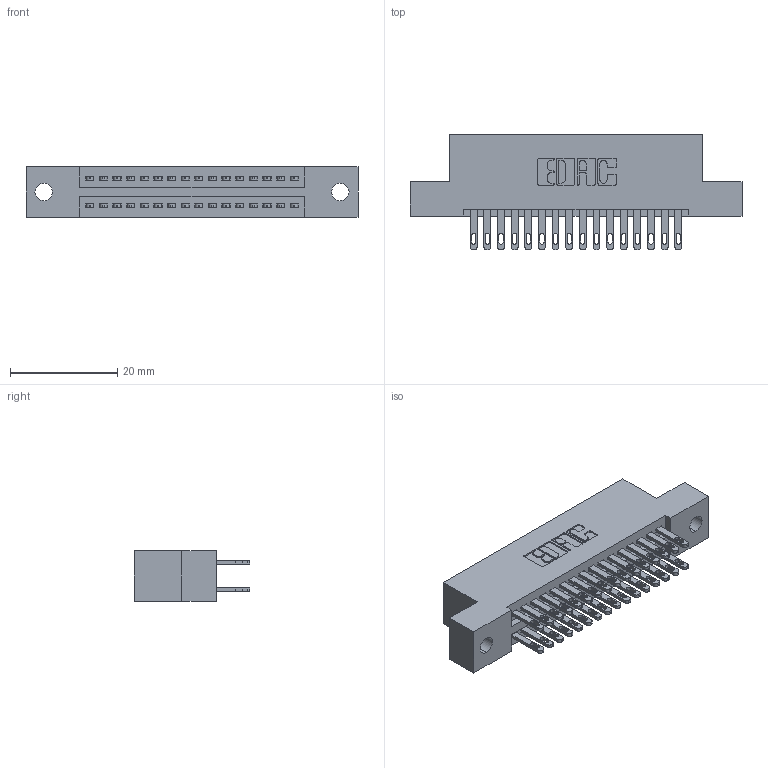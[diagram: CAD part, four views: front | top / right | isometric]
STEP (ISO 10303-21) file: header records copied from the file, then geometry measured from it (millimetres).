
FILE_DESCRIPTION (( 'STEP AP203' ), '1' );
FILE_NAME ('895-032-500-202.STEP', '2020-09-25T19:17:29', ( '' ), ( '' ), 'SwSTEP 2.0', 'SolidWorks 2020', '' );
FILE_SCHEMA (( 'CONFIG_CONTROL_DESIGN' ));
Length unit declared in the file: inch
Products named in the file (3): 845 Part_Flush Mounting Lugs - 0.128 Dia; 895-032-500-202; 345-292-001_345-293-100
Assembly tree (33 placements, depth 2):
  895-032-500-202
    845 Part_Flush Mounting Lugs - 0.128 Dia
    345-292-001_345-293-100  x32
Bounding box: 61.85 x 21.51 x 9.4 mm (x, y, z)
Volume: 5827.8 mm3; surface area: 8164.6 mm2
Topology: 33 solids, 33 shells, 1598 faces, 4853 edges, 3234 vertices
Faces by surface type: plane 944, cylinder 654
Entity records: 15987 total; most frequent: CARTESIAN_POINT 2704, ORIENTED_EDGE 2638, DIRECTION 2419, EDGE_CURVE 1319, VECTOR 1119, LINE 1119, VERTEX_POINT 878, AXIS2_PLACEMENT_3D 650
